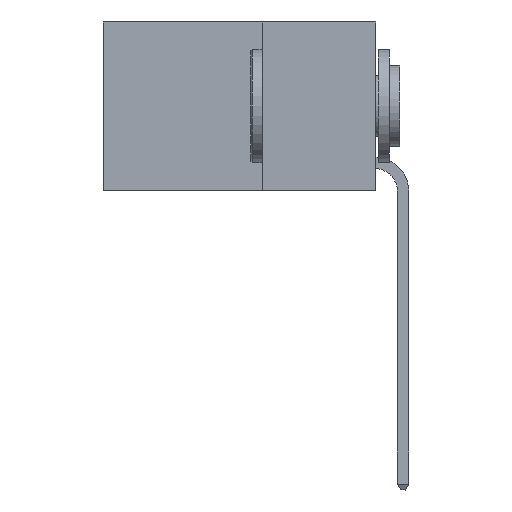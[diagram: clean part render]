
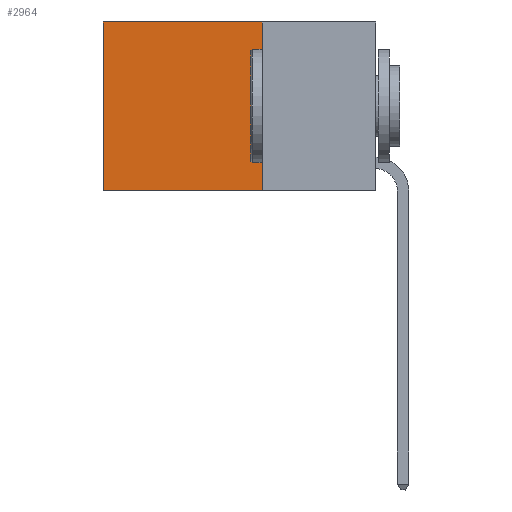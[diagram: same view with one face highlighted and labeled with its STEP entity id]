
A CAD part, left-side view. The second image highlights one B-rep face of the part: STEP entity #2964.
In plain terms, the highlighted planar face has unit normal (-1, 0, 0).
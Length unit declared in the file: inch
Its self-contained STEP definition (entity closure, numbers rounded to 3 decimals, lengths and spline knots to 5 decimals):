
#292 = CARTESIAN_POINT ( 'NONE',  ( 0.2625, 0.25, 0. ) ) ;
#569 = CARTESIAN_POINT ( 'NONE',  ( 0.2625, 0.25, -0.37 ) ) ;
#1445 = PLANE ( 'NONE',  #12066 ) ;
#1918 = ORIENTED_EDGE ( 'NONE', *, *, #16681, .F. ) ;
#2212 = LINE ( 'NONE', #11732, #7385 ) ;
#2964 = ADVANCED_FACE ( 'NONE', ( #4220 ), #1445, .F. ) ;
#3036 = VECTOR ( 'NONE', #14166, 39.37008 ) ;
#3341 = VECTOR ( 'NONE', #19522, 39.37008 ) ;
#3425 = DIRECTION ( 'NONE',  ( 0., 0., -1. ) ) ;
#4220 = FACE_OUTER_BOUND ( 'NONE', #13674, .T. ) ;
#7385 = VECTOR ( 'NONE', #7865, 39.37008 ) ;
#7864 = LINE ( 'NONE', #292, #3341 ) ;
#7865 = DIRECTION ( 'NONE',  ( 0., 1., 0. ) ) ;
#7954 = VERTEX_POINT ( 'NONE', #22830 ) ;
#8787 = VECTOR ( 'NONE', #18061, 39.37008 ) ;
#11115 = CARTESIAN_POINT ( 'NONE',  ( 0.2625, 0.25, 0. ) ) ;
#11252 = EDGE_CURVE ( 'NONE', #14320, #7954, #13901, .T. ) ;
#11732 = CARTESIAN_POINT ( 'NONE',  ( 0.2625, 0.25, 0. ) ) ;
#11780 = VERTEX_POINT ( 'NONE', #19473 ) ;
#12066 = AXIS2_PLACEMENT_3D ( 'NONE', #11115, #18726, #3425 ) ;
#12251 = CARTESIAN_POINT ( 'NONE',  ( 0.2625, 0.6, 0. ) ) ;
#13674 = EDGE_LOOP ( 'NONE', ( #23575, #1918, #19439, #17829 ) ) ;
#13901 = LINE ( 'NONE', #12251, #8787 ) ;
#14050 = EDGE_CURVE ( 'NONE', #24368, #14320, #2212, .T. ) ;
#14166 = DIRECTION ( 'NONE',  ( 0., 1., 0. ) ) ;
#14320 = VERTEX_POINT ( 'NONE', #18202 ) ;
#16681 = EDGE_CURVE ( 'NONE', #11780, #7954, #22811, .T. ) ;
#17829 = ORIENTED_EDGE ( 'NONE', *, *, #14050, .T. ) ;
#18061 = DIRECTION ( 'NONE',  ( 0., 0., -1. ) ) ;
#18202 = CARTESIAN_POINT ( 'NONE',  ( 0.2625, 0.6, 0. ) ) ;
#18726 = DIRECTION ( 'NONE',  ( 1., 0., 0. ) ) ;
#19439 = ORIENTED_EDGE ( 'NONE', *, *, #23965, .F. ) ;
#19473 = CARTESIAN_POINT ( 'NONE',  ( 0.2625, 0.25, -0.37 ) ) ;
#19522 = DIRECTION ( 'NONE',  ( 0., 0., -1. ) ) ;
#22811 = LINE ( 'NONE', #569, #3036 ) ;
#22830 = CARTESIAN_POINT ( 'NONE',  ( 0.2625, 0.6, -0.37 ) ) ;
#23575 = ORIENTED_EDGE ( 'NONE', *, *, #11252, .T. ) ;
#23965 = EDGE_CURVE ( 'NONE', #24368, #11780, #7864, .T. ) ;
#24368 = VERTEX_POINT ( 'NONE', #24452 ) ;
#24452 = CARTESIAN_POINT ( 'NONE',  ( 0.2625, 0.25, 0. ) ) ;
